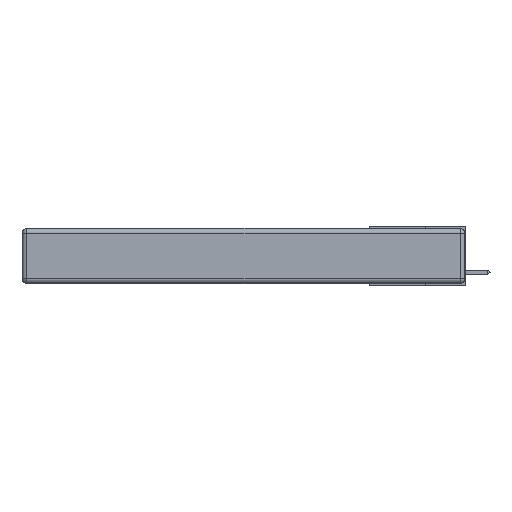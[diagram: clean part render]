
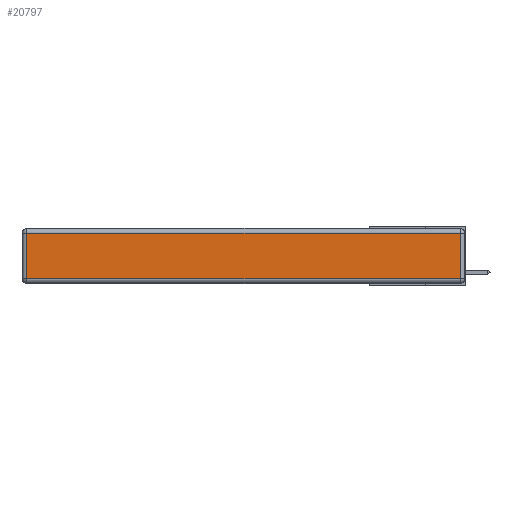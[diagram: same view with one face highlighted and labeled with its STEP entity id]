
A CAD part, left-side view. The second image highlights one B-rep face of the part: STEP entity #20797.
In plain terms, the highlighted planar face has unit normal (-1, 0, 0).
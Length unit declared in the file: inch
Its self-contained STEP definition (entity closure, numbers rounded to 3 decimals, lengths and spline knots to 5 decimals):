
#2231 = LINE ( 'NONE', #9748, #15100 ) ;
#2898 = PLANE ( 'NONE',  #11257 ) ;
#4647 = CARTESIAN_POINT ( 'NONE',  ( 0., 2.75, -0.03 ) ) ;
#5000 = EDGE_LOOP ( 'NONE', ( #8586, #9193, #20910, #15932 ) ) ;
#5043 = EDGE_CURVE ( 'NONE', #19938, #23691, #2231, .T. ) ;
#5451 = CARTESIAN_POINT ( 'NONE',  ( 0., 2.72, -0.313 ) ) ;
#5506 = VECTOR ( 'NONE', #10578, 39.37008 ) ;
#6677 = CARTESIAN_POINT ( 'NONE',  ( 0., 0., -0.343 ) ) ;
#8586 = ORIENTED_EDGE ( 'NONE', *, *, #24121, .T. ) ;
#9193 = ORIENTED_EDGE ( 'NONE', *, *, #12947, .T. ) ;
#9748 = CARTESIAN_POINT ( 'NONE',  ( 0., 2.72, -0.343 ) ) ;
#10578 = DIRECTION ( 'NONE',  ( 0., 0., 1. ) ) ;
#11033 = VERTEX_POINT ( 'NONE', #12644 ) ;
#11257 = AXIS2_PLACEMENT_3D ( 'NONE', #6677, #25138, #12860 ) ;
#12005 = LINE ( 'NONE', #4647, #26195 ) ;
#12644 = CARTESIAN_POINT ( 'NONE',  ( 0., 0.03, -0.313 ) ) ;
#12860 = DIRECTION ( 'NONE',  ( 0., 0., 1. ) ) ;
#12947 = EDGE_CURVE ( 'NONE', #11033, #26356, #16454, .T. ) ;
#15100 = VECTOR ( 'NONE', #23273, 39.37008 ) ;
#15932 = ORIENTED_EDGE ( 'NONE', *, *, #5043, .T. ) ;
#16454 = LINE ( 'NONE', #22955, #5506 ) ;
#17479 = EDGE_CURVE ( 'NONE', #26356, #19938, #12005, .T. ) ;
#17741 = DIRECTION ( 'NONE',  ( 0., -1., 0. ) ) ;
#18502 = VECTOR ( 'NONE', #17741, 39.37008 ) ;
#19048 = DIRECTION ( 'NONE',  ( 0., 1., 0. ) ) ;
#19544 = CARTESIAN_POINT ( 'NONE',  ( 0., 0., -0.313 ) ) ;
#19938 = VERTEX_POINT ( 'NONE', #26347 ) ;
#20797 = ADVANCED_FACE ( 'NONE', ( #22807 ), #2898, .T. ) ;
#20910 = ORIENTED_EDGE ( 'NONE', *, *, #17479, .T. ) ;
#22491 = CARTESIAN_POINT ( 'NONE',  ( 0., 0.03, -0.03 ) ) ;
#22807 = FACE_OUTER_BOUND ( 'NONE', #5000, .T. ) ;
#22955 = CARTESIAN_POINT ( 'NONE',  ( 0., 0.03, -0.343 ) ) ;
#23273 = DIRECTION ( 'NONE',  ( 0., 0., -1. ) ) ;
#23628 = LINE ( 'NONE', #19544, #18502 ) ;
#23691 = VERTEX_POINT ( 'NONE', #5451 ) ;
#24121 = EDGE_CURVE ( 'NONE', #23691, #11033, #23628, .T. ) ;
#25138 = DIRECTION ( 'NONE',  ( -1., 0., 0. ) ) ;
#26195 = VECTOR ( 'NONE', #19048, 39.37008 ) ;
#26347 = CARTESIAN_POINT ( 'NONE',  ( 0., 2.72, -0.03 ) ) ;
#26356 = VERTEX_POINT ( 'NONE', #22491 ) ;
